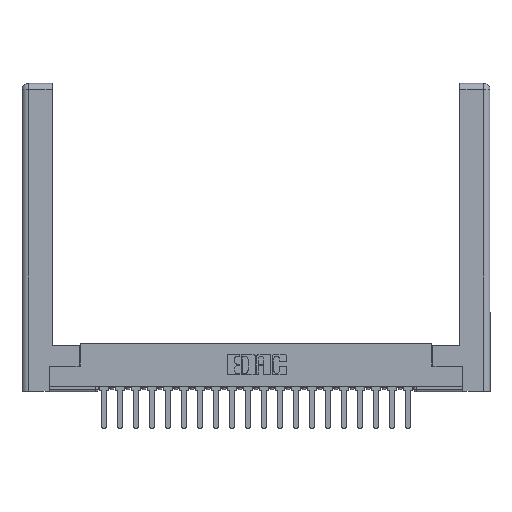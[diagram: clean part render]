
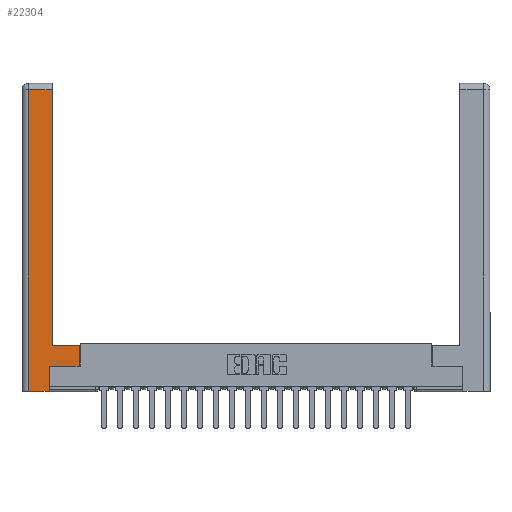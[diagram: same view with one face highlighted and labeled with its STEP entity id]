
A CAD part, top view. The second image highlights one B-rep face of the part: STEP entity #22304.
In plain terms, the highlighted planar face has unit normal (0, 0, 1).
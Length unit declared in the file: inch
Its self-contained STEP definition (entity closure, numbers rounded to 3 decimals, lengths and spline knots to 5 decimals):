
#897 = VERTEX_POINT ( 'NONE', #4955 ) ;
#1338 = LINE ( 'NONE', #8653, #23113 ) ;
#1536 = DIRECTION ( 'NONE',  ( -1., 0., 0. ) ) ;
#1876 = DIRECTION ( 'NONE',  ( 0., 1., 0. ) ) ;
#2284 = FACE_OUTER_BOUND ( 'NONE', #11984, .T. ) ;
#2369 = DIRECTION ( 'NONE',  ( 0., 0., -1. ) ) ;
#2425 = VECTOR ( 'NONE', #19664, 39.37008 ) ;
#2920 = CARTESIAN_POINT ( 'NONE',  ( 0.295, 0.45, 0. ) ) ;
#3511 = CARTESIAN_POINT ( 'NONE',  ( 0.0615, 2.94, 0. ) ) ;
#4761 = EDGE_CURVE ( 'NONE', #20292, #19339, #1338, .T. ) ;
#4769 = LINE ( 'NONE', #2920, #19336 ) ;
#4955 = CARTESIAN_POINT ( 'NONE',  ( 0.265, 0.245, 0. ) ) ;
#6064 = LINE ( 'NONE', #17933, #2425 ) ;
#6068 = CARTESIAN_POINT ( 'NONE',  ( 0.265, 0., 0. ) ) ;
#6111 = CARTESIAN_POINT ( 'NONE',  ( 0.565, 0.245, 0. ) ) ;
#6726 = EDGE_CURVE ( 'NONE', #897, #15518, #22443, .T. ) ;
#6891 = VECTOR ( 'NONE', #1876, 39.37008 ) ;
#6921 = EDGE_CURVE ( 'NONE', #13235, #20832, #13233, .T. ) ;
#7448 = CARTESIAN_POINT ( 'NONE',  ( 0.265, 0., 0. ) ) ;
#7783 = VERTEX_POINT ( 'NONE', #8806 ) ;
#7937 = CARTESIAN_POINT ( 'NONE',  ( 0.295, 2.94, 0. ) ) ;
#8007 = EDGE_CURVE ( 'NONE', #19339, #13235, #18227, .T. ) ;
#8098 = CARTESIAN_POINT ( 'NONE',  ( 0.0615, 0., 0. ) ) ;
#8267 = LINE ( 'NONE', #12564, #6891 ) ;
#8546 = CARTESIAN_POINT ( 'NONE',  ( 0.295, 0.45, 0. ) ) ;
#8653 = CARTESIAN_POINT ( 'NONE',  ( 0.0615, 2.94, 0. ) ) ;
#8806 = CARTESIAN_POINT ( 'NONE',  ( 0.565, 0.45, 0. ) ) ;
#9084 = ORIENTED_EDGE ( 'NONE', *, *, #17223, .T. ) ;
#9270 = ORIENTED_EDGE ( 'NONE', *, *, #8007, .T. ) ;
#9704 = DIRECTION ( 'NONE',  ( -1., 0., 0. ) ) ;
#11001 = EDGE_CURVE ( 'NONE', #15518, #7783, #6064, .T. ) ;
#11043 = CARTESIAN_POINT ( 'NONE',  ( 0.0615, 0., 0. ) ) ;
#11365 = DIRECTION ( 'NONE',  ( 1., 0., 0. ) ) ;
#11984 = EDGE_LOOP ( 'NONE', ( #16834, #14109, #9270, #15431, #9084, #12144, #18148, #15284 ) ) ;
#12039 = DIRECTION ( 'NONE',  ( 0., 1., 0. ) ) ;
#12144 = ORIENTED_EDGE ( 'NONE', *, *, #6726, .T. ) ;
#12288 = EDGE_CURVE ( 'NONE', #20534, #20292, #8267, .T. ) ;
#12507 = AXIS2_PLACEMENT_3D ( 'NONE', #13061, #2369, #20098 ) ;
#12564 = CARTESIAN_POINT ( 'NONE',  ( 0.295, 3., 0. ) ) ;
#12950 = VECTOR ( 'NONE', #22131, 39.37008 ) ;
#13061 = CARTESIAN_POINT ( 'NONE',  ( 0., 0., 0. ) ) ;
#13233 = LINE ( 'NONE', #6068, #14318 ) ;
#13235 = VERTEX_POINT ( 'NONE', #8098 ) ;
#13464 = VECTOR ( 'NONE', #16577, 39.37008 ) ;
#14109 = ORIENTED_EDGE ( 'NONE', *, *, #4761, .T. ) ;
#14318 = VECTOR ( 'NONE', #11365, 39.37008 ) ;
#14864 = CARTESIAN_POINT ( 'NONE',  ( 0.565, 0.245, 0. ) ) ;
#15035 = LINE ( 'NONE', #15070, #20921 ) ;
#15070 = CARTESIAN_POINT ( 'NONE',  ( 0.265, 0.245, 0. ) ) ;
#15284 = ORIENTED_EDGE ( 'NONE', *, *, #22352, .T. ) ;
#15431 = ORIENTED_EDGE ( 'NONE', *, *, #6921, .T. ) ;
#15518 = VERTEX_POINT ( 'NONE', #6111 ) ;
#16577 = DIRECTION ( 'NONE',  ( 0., -1., 0. ) ) ;
#16834 = ORIENTED_EDGE ( 'NONE', *, *, #12288, .T. ) ;
#17223 = EDGE_CURVE ( 'NONE', #20832, #897, #15035, .T. ) ;
#17933 = CARTESIAN_POINT ( 'NONE',  ( 0.565, 0.45, 0. ) ) ;
#18148 = ORIENTED_EDGE ( 'NONE', *, *, #11001, .T. ) ;
#18227 = LINE ( 'NONE', #11043, #13464 ) ;
#19336 = VECTOR ( 'NONE', #9704, 39.37008 ) ;
#19339 = VERTEX_POINT ( 'NONE', #3511 ) ;
#19664 = DIRECTION ( 'NONE',  ( 0., 1., 0. ) ) ;
#20098 = DIRECTION ( 'NONE',  ( -1., 0., 0. ) ) ;
#20292 = VERTEX_POINT ( 'NONE', #7937 ) ;
#20534 = VERTEX_POINT ( 'NONE', #8546 ) ;
#20832 = VERTEX_POINT ( 'NONE', #7448 ) ;
#20921 = VECTOR ( 'NONE', #12039, 39.37008 ) ;
#21798 = PLANE ( 'NONE',  #12507 ) ;
#22131 = DIRECTION ( 'NONE',  ( 1., 0., 0. ) ) ;
#22304 = ADVANCED_FACE ( 'NONE', ( #2284 ), #21798, .F. ) ;
#22352 = EDGE_CURVE ( 'NONE', #7783, #20534, #4769, .T. ) ;
#22443 = LINE ( 'NONE', #14864, #12950 ) ;
#23113 = VECTOR ( 'NONE', #1536, 39.37008 ) ;
